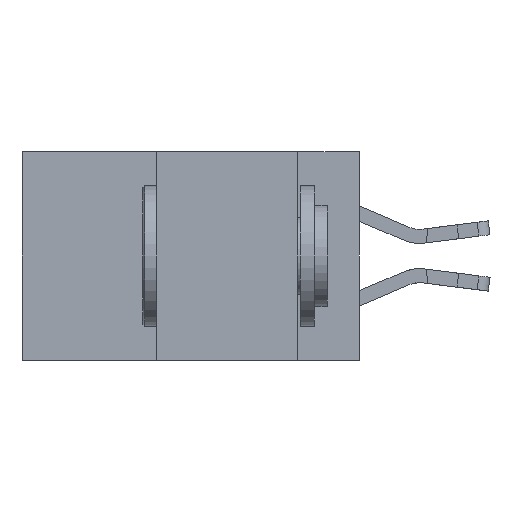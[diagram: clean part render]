
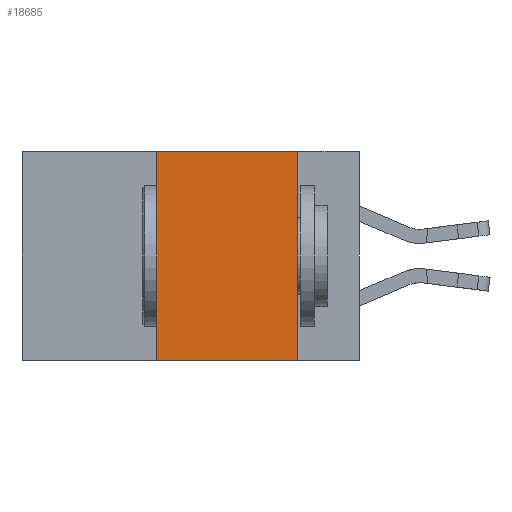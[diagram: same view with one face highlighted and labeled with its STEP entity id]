
A CAD part, left-side view. The second image highlights one B-rep face of the part: STEP entity #18685.
In plain terms, the highlighted planar face has unit normal (-1, 0, 0).
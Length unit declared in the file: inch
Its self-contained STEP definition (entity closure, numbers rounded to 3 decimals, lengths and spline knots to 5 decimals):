
#1118 = LINE ( 'NONE', #3348, #19287 ) ;
#1126 = DIRECTION ( 'NONE',  ( 0., -1., 0. ) ) ;
#1254 = VECTOR ( 'NONE', #10005, 39.37008 ) ;
#1657 = EDGE_CURVE ( 'NONE', #7921, #3944, #21540, .T. ) ;
#1797 = DIRECTION ( 'NONE',  ( 1., 0., 0. ) ) ;
#3348 = CARTESIAN_POINT ( 'NONE',  ( 0., 0.36, 0. ) ) ;
#3944 = VERTEX_POINT ( 'NONE', #4843 ) ;
#4051 = VECTOR ( 'NONE', #1126, 39.37008 ) ;
#4843 = CARTESIAN_POINT ( 'NONE',  ( 0., 0.11, -0.37 ) ) ;
#4950 = LINE ( 'NONE', #17034, #1254 ) ;
#6513 = CARTESIAN_POINT ( 'NONE',  ( 0., 0.6, -0.37 ) ) ;
#7124 = CARTESIAN_POINT ( 'NONE',  ( 0., 0.36, -0.37 ) ) ;
#7247 = CARTESIAN_POINT ( 'NONE',  ( 0., 0.11, 0. ) ) ;
#7644 = CARTESIAN_POINT ( 'NONE',  ( 0., 0.36, 0. ) ) ;
#7759 = ORIENTED_EDGE ( 'NONE', *, *, #14930, .F. ) ;
#7842 = CARTESIAN_POINT ( 'NONE',  ( 0., 0.11, 0. ) ) ;
#7921 = VERTEX_POINT ( 'NONE', #7842 ) ;
#8865 = ORIENTED_EDGE ( 'NONE', *, *, #18443, .T. ) ;
#10005 = DIRECTION ( 'NONE',  ( 0., -1., 0. ) ) ;
#10814 = ORIENTED_EDGE ( 'NONE', *, *, #1657, .F. ) ;
#11964 = VERTEX_POINT ( 'NONE', #7124 ) ;
#12325 = VECTOR ( 'NONE', #22472, 39.37008 ) ;
#12342 = EDGE_CURVE ( 'NONE', #21393, #7921, #4950, .T. ) ;
#12614 = CARTESIAN_POINT ( 'NONE',  ( 0., 0.6, 0. ) ) ;
#13599 = LINE ( 'NONE', #6513, #4051 ) ;
#14167 = DIRECTION ( 'NONE',  ( 0., 0., 1. ) ) ;
#14377 = DIRECTION ( 'NONE',  ( 0., 0., -1. ) ) ;
#14930 = EDGE_CURVE ( 'NONE', #11964, #21393, #1118, .T. ) ;
#15007 = AXIS2_PLACEMENT_3D ( 'NONE', #12614, #1797, #14377 ) ;
#16649 = ORIENTED_EDGE ( 'NONE', *, *, #12342, .F. ) ;
#16872 = FACE_OUTER_BOUND ( 'NONE', #18123, .T. ) ;
#17034 = CARTESIAN_POINT ( 'NONE',  ( 0., 0.6, 0. ) ) ;
#18123 = EDGE_LOOP ( 'NONE', ( #10814, #16649, #7759, #8865 ) ) ;
#18443 = EDGE_CURVE ( 'NONE', #11964, #3944, #13599, .T. ) ;
#18685 = ADVANCED_FACE ( 'NONE', ( #16872 ), #19570, .F. ) ;
#19287 = VECTOR ( 'NONE', #14167, 39.37008 ) ;
#19570 = PLANE ( 'NONE',  #15007 ) ;
#21393 = VERTEX_POINT ( 'NONE', #7644 ) ;
#21540 = LINE ( 'NONE', #7247, #12325 ) ;
#22472 = DIRECTION ( 'NONE',  ( 0., 0., -1. ) ) ;
